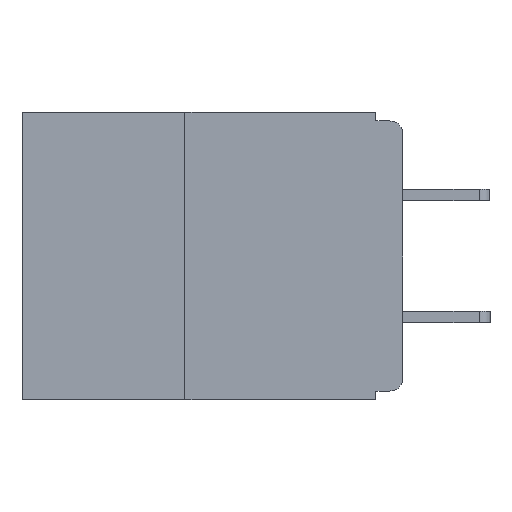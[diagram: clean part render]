
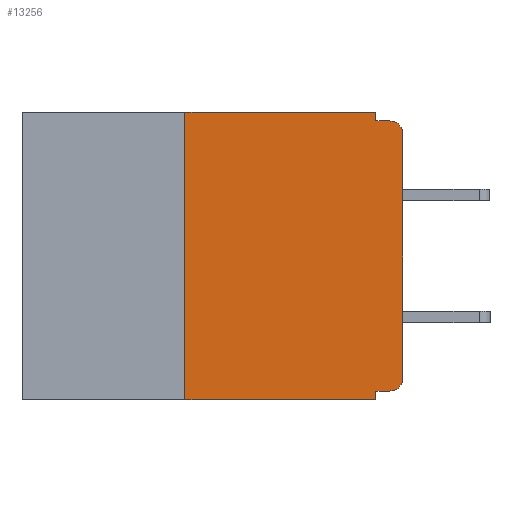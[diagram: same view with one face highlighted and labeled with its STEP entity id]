
A CAD part, left-side view. The second image highlights one B-rep face of the part: STEP entity #13256.
In plain terms, the highlighted planar face has unit normal (-1, 0, 0).
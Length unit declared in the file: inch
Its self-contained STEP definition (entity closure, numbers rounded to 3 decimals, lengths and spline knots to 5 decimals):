
#107 = DIRECTION ( 'NONE',  ( -1., 0., 0. ) ) ;
#440 = CARTESIAN_POINT ( 'NONE',  ( 0., 0., -0.025 ) ) ;
#615 = DIRECTION ( 'NONE',  ( 0., -1., 0. ) ) ;
#867 = DIRECTION ( 'NONE',  ( 0., 0., -1. ) ) ;
#1216 = LINE ( 'NONE', #11811, #15040 ) ;
#2929 = AXIS2_PLACEMENT_3D ( 'NONE', #16675, #107, #19411 ) ;
#3020 = DIRECTION ( 'NONE',  ( 0., -1., 0. ) ) ;
#3389 = CARTESIAN_POINT ( 'NONE',  ( 0., 0., -0.32 ) ) ;
#3449 = LINE ( 'NONE', #6115, #18074 ) ;
#3557 = CARTESIAN_POINT ( 'NONE',  ( 0., 0.437, 0. ) ) ;
#4820 = EDGE_CURVE ( 'NONE', #22447, #14673, #23727, .T. ) ;
#5069 = CARTESIAN_POINT ( 'NONE',  ( 0., 0.031, -0.32 ) ) ;
#5458 = EDGE_CURVE ( 'NONE', #19737, #22447, #15101, .T. ) ;
#6115 = CARTESIAN_POINT ( 'NONE',  ( 0., 0.031, 0. ) ) ;
#6204 = ORIENTED_EDGE ( 'NONE', *, *, #19911, .F. ) ;
#6731 = CARTESIAN_POINT ( 'NONE',  ( 0., 0.031, -0.33 ) ) ;
#6997 = CARTESIAN_POINT ( 'NONE',  ( 0., 0.015, -0.32 ) ) ;
#7585 = DIRECTION ( 'NONE',  ( 0., 0., 1. ) ) ;
#8109 = LINE ( 'NONE', #19454, #34955 ) ;
#8563 = CARTESIAN_POINT ( 'NONE',  ( 0., 0.031, -0.01 ) ) ;
#8815 = DIRECTION ( 'NONE',  ( -1., 0., 0. ) ) ;
#9276 = ORIENTED_EDGE ( 'NONE', *, *, #5458, .T. ) ;
#9900 = AXIS2_PLACEMENT_3D ( 'NONE', #29948, #13748, #32498 ) ;
#10082 = VECTOR ( 'NONE', #7585, 39.37008 ) ;
#11029 = PLANE ( 'NONE',  #9900 ) ;
#11334 = EDGE_LOOP ( 'NONE', ( #9276, #32410, #12691, #19942, #6204, #24240, #25920, #20418, #27592, #29243 ) ) ;
#11691 = CIRCLE ( 'NONE', #18091, 0.015 ) ;
#11811 = CARTESIAN_POINT ( 'NONE',  ( 0., 0.031, -0.33 ) ) ;
#11859 = LINE ( 'NONE', #3389, #25492 ) ;
#12193 = EDGE_CURVE ( 'NONE', #14474, #19737, #11691, .T. ) ;
#12230 = EDGE_CURVE ( 'NONE', #17791, #27194, #3449, .T. ) ;
#12691 = ORIENTED_EDGE ( 'NONE', *, *, #18363, .F. ) ;
#13256 = ADVANCED_FACE ( 'NONE', ( #33406 ), #11029, .F. ) ;
#13748 = DIRECTION ( 'NONE',  ( 1., 0., 0. ) ) ;
#14418 = CARTESIAN_POINT ( 'NONE',  ( 0., 0., -0.01 ) ) ;
#14474 = VERTEX_POINT ( 'NONE', #6997 ) ;
#14673 = VERTEX_POINT ( 'NONE', #26938 ) ;
#15040 = VECTOR ( 'NONE', #867, 39.37008 ) ;
#15101 = LINE ( 'NONE', #30069, #29472 ) ;
#15736 = CARTESIAN_POINT ( 'NONE',  ( 0., 0.25, -0.33 ) ) ;
#16546 = CARTESIAN_POINT ( 'NONE',  ( 0., 0., -0.305 ) ) ;
#16675 = CARTESIAN_POINT ( 'NONE',  ( 0., 0.015, -0.025 ) ) ;
#17274 = DIRECTION ( 'NONE',  ( 0., -1., 0. ) ) ;
#17791 = VERTEX_POINT ( 'NONE', #25645 ) ;
#18074 = VECTOR ( 'NONE', #22547, 39.37008 ) ;
#18078 = VERTEX_POINT ( 'NONE', #5069 ) ;
#18091 = AXIS2_PLACEMENT_3D ( 'NONE', #25161, #8815, #27848 ) ;
#18363 = EDGE_CURVE ( 'NONE', #27194, #14673, #21067, .T. ) ;
#19411 = DIRECTION ( 'NONE',  ( 0., 0., -1. ) ) ;
#19454 = CARTESIAN_POINT ( 'NONE',  ( 0., 0.437, -0.33 ) ) ;
#19737 = VERTEX_POINT ( 'NONE', #16546 ) ;
#19911 = EDGE_CURVE ( 'NONE', #27565, #17791, #26494, .T. ) ;
#19942 = ORIENTED_EDGE ( 'NONE', *, *, #12230, .F. ) ;
#20418 = ORIENTED_EDGE ( 'NONE', *, *, #25451, .F. ) ;
#21067 = LINE ( 'NONE', #14418, #34267 ) ;
#21210 = VERTEX_POINT ( 'NONE', #6731 ) ;
#22447 = VERTEX_POINT ( 'NONE', #440 ) ;
#22547 = DIRECTION ( 'NONE',  ( 0., 0., -1. ) ) ;
#22978 = CARTESIAN_POINT ( 'NONE',  ( 0., 0.25, -0.33 ) ) ;
#23727 = CIRCLE ( 'NONE', #2929, 0.015 ) ;
#24240 = ORIENTED_EDGE ( 'NONE', *, *, #33533, .F. ) ;
#24305 = CARTESIAN_POINT ( 'NONE',  ( 0., 0.25, 0. ) ) ;
#25161 = CARTESIAN_POINT ( 'NONE',  ( 0., 0.015, -0.305 ) ) ;
#25451 = EDGE_CURVE ( 'NONE', #18078, #21210, #1216, .T. ) ;
#25492 = VECTOR ( 'NONE', #33186, 39.37008 ) ;
#25645 = CARTESIAN_POINT ( 'NONE',  ( 0., 0.031, 0. ) ) ;
#25920 = ORIENTED_EDGE ( 'NONE', *, *, #26584, .T. ) ;
#26093 = VERTEX_POINT ( 'NONE', #22978 ) ;
#26494 = LINE ( 'NONE', #3557, #33398 ) ;
#26584 = EDGE_CURVE ( 'NONE', #26093, #21210, #8109, .T. ) ;
#26938 = CARTESIAN_POINT ( 'NONE',  ( 0., 0.015, -0.01 ) ) ;
#27194 = VERTEX_POINT ( 'NONE', #8563 ) ;
#27565 = VERTEX_POINT ( 'NONE', #24305 ) ;
#27592 = ORIENTED_EDGE ( 'NONE', *, *, #32625, .F. ) ;
#27848 = DIRECTION ( 'NONE',  ( 0., 0., -1. ) ) ;
#29243 = ORIENTED_EDGE ( 'NONE', *, *, #12193, .T. ) ;
#29472 = VECTOR ( 'NONE', #32628, 39.37008 ) ;
#29948 = CARTESIAN_POINT ( 'NONE',  ( 0., 0.437, 0. ) ) ;
#30069 = CARTESIAN_POINT ( 'NONE',  ( 0., 0., 0. ) ) ;
#30794 = LINE ( 'NONE', #15736, #10082 ) ;
#32410 = ORIENTED_EDGE ( 'NONE', *, *, #4820, .T. ) ;
#32498 = DIRECTION ( 'NONE',  ( 0., 0., -1. ) ) ;
#32625 = EDGE_CURVE ( 'NONE', #14474, #18078, #11859, .T. ) ;
#32628 = DIRECTION ( 'NONE',  ( 0., 0., 1. ) ) ;
#33186 = DIRECTION ( 'NONE',  ( 0., 1., 0. ) ) ;
#33398 = VECTOR ( 'NONE', #17274, 39.37008 ) ;
#33406 = FACE_OUTER_BOUND ( 'NONE', #11334, .T. ) ;
#33533 = EDGE_CURVE ( 'NONE', #26093, #27565, #30794, .T. ) ;
#34267 = VECTOR ( 'NONE', #615, 39.37008 ) ;
#34955 = VECTOR ( 'NONE', #3020, 39.37008 ) ;
